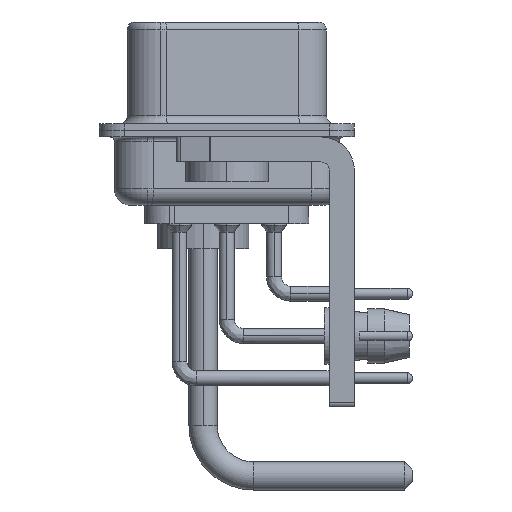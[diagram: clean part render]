
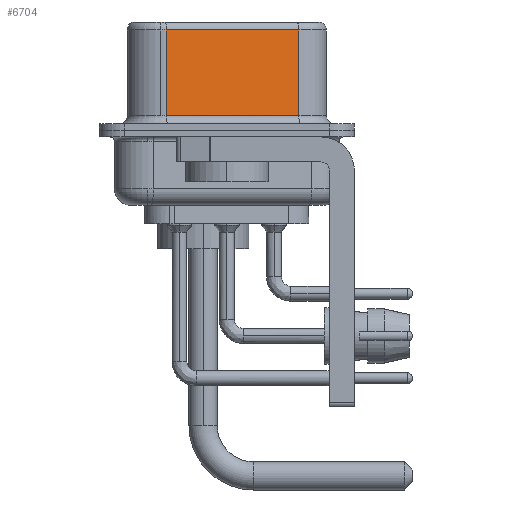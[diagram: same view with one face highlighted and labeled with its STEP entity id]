
A CAD part, left-side view. The second image highlights one B-rep face of the part: STEP entity #6704.
In plain terms, the highlighted planar face has unit normal (-0.985, -0.174, 0).
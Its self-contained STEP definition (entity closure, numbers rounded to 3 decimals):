
#331 = VECTOR ( 'NONE', #7886, 1000. ) ;
#503 = VERTEX_POINT ( 'NONE', #4889 ) ;
#869 = EDGE_CURVE ( 'NONE', #16711, #503, #4275, .T. ) ;
#3875 = CARTESIAN_POINT ( 'NONE',  ( 5.132, -4.322, 6.02 ) ) ;
#4275 = LINE ( 'NONE', #3875, #23376 ) ;
#4889 = CARTESIAN_POINT ( 'NONE',  ( 3.73, 3.628, 6.02 ) ) ;
#6128 = DIRECTION ( 'NONE',  ( 0.985, 0.174, 0. ) ) ;
#6292 = EDGE_CURVE ( 'NONE', #16711, #7432, #27925, .T. ) ;
#6704 = ADVANCED_FACE ( 'NONE', ( #35968 ), #9047, .F. ) ;
#6817 = ORIENTED_EDGE ( 'NONE', *, *, #869, .T. ) ;
#7432 = VERTEX_POINT ( 'NONE', #36602 ) ;
#7886 = DIRECTION ( 'NONE',  ( 0., 0., -1. ) ) ;
#9047 = PLANE ( 'NONE',  #13950 ) ;
#9853 = CARTESIAN_POINT ( 'NONE',  ( 5.132, -4.322, 6.52 ) ) ;
#10815 = LINE ( 'NONE', #34809, #331 ) ;
#11792 = CARTESIAN_POINT ( 'NONE',  ( 5.132, -4.322, 6.52 ) ) ;
#12419 = ORIENTED_EDGE ( 'NONE', *, *, #37864, .T. ) ;
#12972 = VERTEX_POINT ( 'NONE', #25755 ) ;
#13345 = EDGE_LOOP ( 'NONE', ( #33489, #6817, #12419, #34924 ) ) ;
#13950 = AXIS2_PLACEMENT_3D ( 'NONE', #11792, #6128, #18080 ) ;
#14717 = VECTOR ( 'NONE', #35322, 1000. ) ;
#16234 = DIRECTION ( 'NONE',  ( -0.174, 0.985, 0. ) ) ;
#16711 = VERTEX_POINT ( 'NONE', #38721 ) ;
#18080 = DIRECTION ( 'NONE',  ( -0.174, 0.985, 0. ) ) ;
#23329 = EDGE_CURVE ( 'NONE', #12972, #7432, #38072, .T. ) ;
#23330 = CARTESIAN_POINT ( 'NONE',  ( 5.132, -4.322, 0.9 ) ) ;
#23376 = VECTOR ( 'NONE', #16234, 1000. ) ;
#25755 = CARTESIAN_POINT ( 'NONE',  ( 3.73, 3.628, 0.9 ) ) ;
#27925 = LINE ( 'NONE', #9853, #32856 ) ;
#31469 = DIRECTION ( 'NONE',  ( 0., 0., -1. ) ) ;
#32856 = VECTOR ( 'NONE', #31469, 1000. ) ;
#33489 = ORIENTED_EDGE ( 'NONE', *, *, #6292, .F. ) ;
#34809 = CARTESIAN_POINT ( 'NONE',  ( 3.73, 3.628, 6.52 ) ) ;
#34924 = ORIENTED_EDGE ( 'NONE', *, *, #23329, .T. ) ;
#35322 = DIRECTION ( 'NONE',  ( 0.174, -0.985, 0. ) ) ;
#35968 = FACE_OUTER_BOUND ( 'NONE', #13345, .T. ) ;
#36602 = CARTESIAN_POINT ( 'NONE',  ( 5.132, -4.322, 0.9 ) ) ;
#37864 = EDGE_CURVE ( 'NONE', #503, #12972, #10815, .T. ) ;
#38072 = LINE ( 'NONE', #23330, #14717 ) ;
#38721 = CARTESIAN_POINT ( 'NONE',  ( 5.132, -4.322, 6.02 ) ) ;
